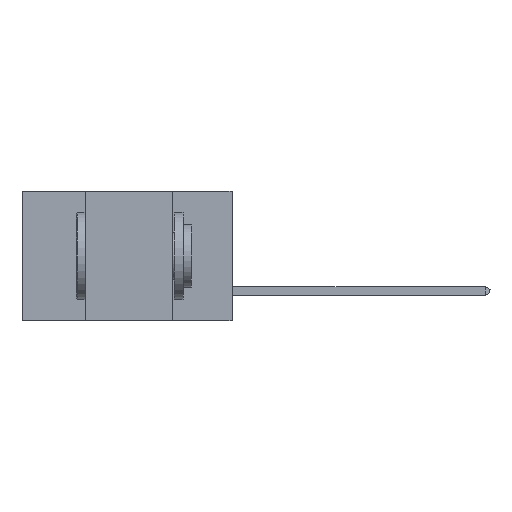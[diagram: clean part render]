
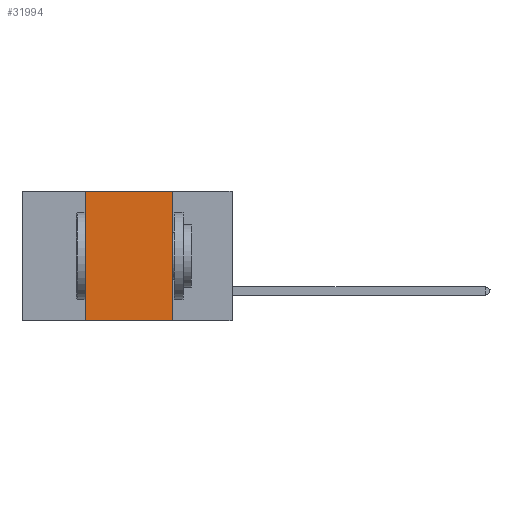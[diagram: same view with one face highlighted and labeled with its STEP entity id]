
A CAD part, left-side view. The second image highlights one B-rep face of the part: STEP entity #31994.
In plain terms, the highlighted planar face has unit normal (-1, 0, 0).
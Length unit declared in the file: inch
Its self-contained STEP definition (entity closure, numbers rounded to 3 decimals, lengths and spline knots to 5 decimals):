
#429 = PLANE ( 'NONE',  #33503 ) ;
#3881 = EDGE_CURVE ( 'NONE', #6195, #19591, #26850, .T. ) ;
#4172 = LINE ( 'NONE', #29575, #39747 ) ;
#5840 = FACE_OUTER_BOUND ( 'NONE', #31846, .T. ) ;
#6195 = VERTEX_POINT ( 'NONE', #34057 ) ;
#6433 = DIRECTION ( 'NONE',  ( 0., 0., 1. ) ) ;
#6809 = VECTOR ( 'NONE', #30792, 39.37008 ) ;
#7108 = DIRECTION ( 'NONE',  ( 0., 0., -1. ) ) ;
#12211 = ORIENTED_EDGE ( 'NONE', *, *, #24673, .F. ) ;
#12372 = CARTESIAN_POINT ( 'NONE',  ( 0., 0.42, -0.37 ) ) ;
#13565 = ORIENTED_EDGE ( 'NONE', *, *, #3881, .F. ) ;
#14323 = CARTESIAN_POINT ( 'NONE',  ( 0., 0.17, 0. ) ) ;
#16340 = DIRECTION ( 'NONE',  ( 0., -1., 0. ) ) ;
#16707 = VECTOR ( 'NONE', #18370, 39.37008 ) ;
#18240 = VECTOR ( 'NONE', #16340, 39.37008 ) ;
#18370 = DIRECTION ( 'NONE',  ( 0., -1., 0. ) ) ;
#18804 = ORIENTED_EDGE ( 'NONE', *, *, #39481, .F. ) ;
#19591 = VERTEX_POINT ( 'NONE', #25701 ) ;
#19885 = CARTESIAN_POINT ( 'NONE',  ( 0., 0.6, 0. ) ) ;
#23416 = DIRECTION ( 'NONE',  ( 1., 0., 0. ) ) ;
#24673 = EDGE_CURVE ( 'NONE', #19591, #27615, #25084, .T. ) ;
#25084 = LINE ( 'NONE', #14323, #6809 ) ;
#25701 = CARTESIAN_POINT ( 'NONE',  ( 0., 0.17, 0. ) ) ;
#26850 = LINE ( 'NONE', #19885, #18240 ) ;
#26958 = CARTESIAN_POINT ( 'NONE',  ( 0., 0.6, 0. ) ) ;
#27615 = VERTEX_POINT ( 'NONE', #38486 ) ;
#28045 = EDGE_CURVE ( 'NONE', #41406, #27615, #28915, .T. ) ;
#28915 = LINE ( 'NONE', #31683, #16707 ) ;
#29575 = CARTESIAN_POINT ( 'NONE',  ( 0., 0.42, 0. ) ) ;
#30792 = DIRECTION ( 'NONE',  ( 0., 0., -1. ) ) ;
#31683 = CARTESIAN_POINT ( 'NONE',  ( 0., 0.6, -0.37 ) ) ;
#31846 = EDGE_LOOP ( 'NONE', ( #12211, #13565, #18804, #37871 ) ) ;
#31994 = ADVANCED_FACE ( 'NONE', ( #5840 ), #429, .F. ) ;
#33503 = AXIS2_PLACEMENT_3D ( 'NONE', #26958, #23416, #7108 ) ;
#34057 = CARTESIAN_POINT ( 'NONE',  ( 0., 0.42, 0. ) ) ;
#37871 = ORIENTED_EDGE ( 'NONE', *, *, #28045, .T. ) ;
#38486 = CARTESIAN_POINT ( 'NONE',  ( 0., 0.17, -0.37 ) ) ;
#39481 = EDGE_CURVE ( 'NONE', #41406, #6195, #4172, .T. ) ;
#39747 = VECTOR ( 'NONE', #6433, 39.37008 ) ;
#41406 = VERTEX_POINT ( 'NONE', #12372 ) ;
